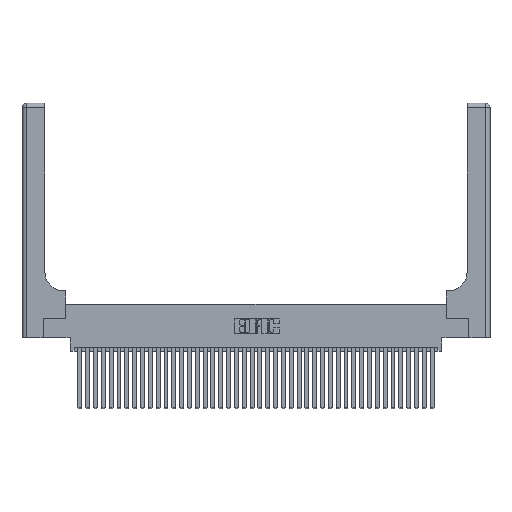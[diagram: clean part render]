
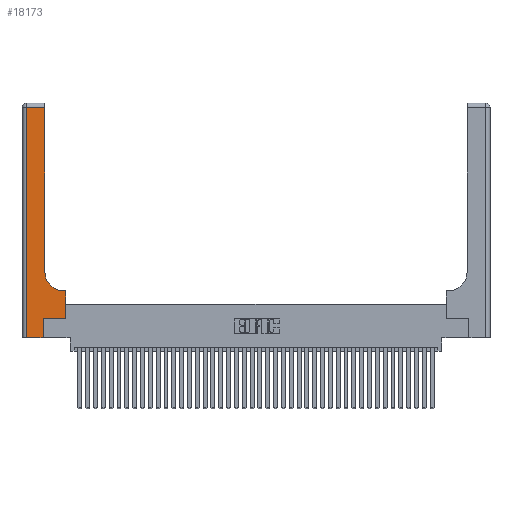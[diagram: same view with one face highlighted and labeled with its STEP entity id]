
A CAD part, top view. The second image highlights one B-rep face of the part: STEP entity #18173.
In plain terms, the highlighted planar face has unit normal (0, 0, 1).
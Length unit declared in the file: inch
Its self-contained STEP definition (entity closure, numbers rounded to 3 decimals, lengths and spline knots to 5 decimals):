
#186 = DIRECTION ( 'NONE',  ( -1., 0., 0. ) ) ;
#487 = CARTESIAN_POINT ( 'NONE',  ( 0.2915, 2.94, 0.37 ) ) ;
#1259 = VECTOR ( 'NONE', #11023, 39.37008 ) ;
#1496 = CARTESIAN_POINT ( 'NONE',  ( 0.2915, 0.6, 0.37 ) ) ;
#1696 = ORIENTED_EDGE ( 'NONE', *, *, #18250, .T. ) ;
#3113 = VECTOR ( 'NONE', #39461, 39.37008 ) ;
#3179 = VERTEX_POINT ( 'NONE', #7423 ) ;
#3605 = CARTESIAN_POINT ( 'NONE',  ( 0., 2.94, 0.37 ) ) ;
#3863 = LINE ( 'NONE', #4977, #11738 ) ;
#4977 = CARTESIAN_POINT ( 'NONE',  ( 0.269, 0., 0.37 ) ) ;
#5145 = CARTESIAN_POINT ( 'NONE',  ( 0.269, 0., 0.37 ) ) ;
#5342 = CARTESIAN_POINT ( 'NONE',  ( 0.5585, 0.6, 0.37 ) ) ;
#5347 = VERTEX_POINT ( 'NONE', #36318 ) ;
#5669 = AXIS2_PLACEMENT_3D ( 'NONE', #19370, #12613, #28831 ) ;
#6609 = DIRECTION ( 'NONE',  ( 1., 0., 0. ) ) ;
#6881 = EDGE_CURVE ( 'NONE', #18473, #3179, #17303, .T. ) ;
#7340 = DIRECTION ( 'NONE',  ( 0., 1., 0. ) ) ;
#7350 = CARTESIAN_POINT ( 'NONE',  ( 0.06, 0., 0.37 ) ) ;
#7379 = CARTESIAN_POINT ( 'NONE',  ( 0.269, 0.25, 0.37 ) ) ;
#7423 = CARTESIAN_POINT ( 'NONE',  ( 0.5585, 0.25, 0.37 ) ) ;
#7628 = LINE ( 'NONE', #20832, #1259 ) ;
#7651 = DIRECTION ( 'NONE',  ( -1., 0., 0. ) ) ;
#8691 = ORIENTED_EDGE ( 'NONE', *, *, #23717, .T. ) ;
#9276 = ORIENTED_EDGE ( 'NONE', *, *, #30700, .T. ) ;
#10074 = ORIENTED_EDGE ( 'NONE', *, *, #35673, .T. ) ;
#10418 = EDGE_CURVE ( 'NONE', #5347, #30091, #19986, .T. ) ;
#11023 = DIRECTION ( 'NONE',  ( 1., 0., 0. ) ) ;
#11505 = LINE ( 'NONE', #1496, #15518 ) ;
#11738 = VECTOR ( 'NONE', #36791, 39.37008 ) ;
#12613 = DIRECTION ( 'NONE',  ( 0., 0., -1. ) ) ;
#14313 = VECTOR ( 'NONE', #186, 39.37008 ) ;
#14418 = VERTEX_POINT ( 'NONE', #25657 ) ;
#15518 = VECTOR ( 'NONE', #7651, 39.37008 ) ;
#15998 = CARTESIAN_POINT ( 'NONE',  ( 0.269, 0.25, 0.37 ) ) ;
#17303 = LINE ( 'NONE', #15998, #22685 ) ;
#17539 = CARTESIAN_POINT ( 'NONE',  ( 0.2915, 0.85, 0.37 ) ) ;
#18173 = ADVANCED_FACE ( 'NONE', ( #25512 ), #30043, .F. ) ;
#18250 = EDGE_CURVE ( 'NONE', #36954, #18473, #3863, .T. ) ;
#18264 = LINE ( 'NONE', #3605, #14313 ) ;
#18473 = VERTEX_POINT ( 'NONE', #7379 ) ;
#18746 = EDGE_LOOP ( 'NONE', ( #9276, #8691, #24765, #40462, #1696, #39995, #23211, #10074, #25572 ) ) ;
#19227 = AXIS2_PLACEMENT_3D ( 'NONE', #33217, #23860, #27174 ) ;
#19370 = CARTESIAN_POINT ( 'NONE',  ( 0.5415, 0.85, 0.37 ) ) ;
#19986 = CIRCLE ( 'NONE', #5669, 0.25 ) ;
#20832 = CARTESIAN_POINT ( 'NONE',  ( 0., 0., 0.37 ) ) ;
#22685 = VECTOR ( 'NONE', #6609, 39.37008 ) ;
#23075 = CARTESIAN_POINT ( 'NONE',  ( 0.5585, 0.25, 0.37 ) ) ;
#23211 = ORIENTED_EDGE ( 'NONE', *, *, #25624, .T. ) ;
#23504 = CARTESIAN_POINT ( 'NONE',  ( 0.06, 3., 0.37 ) ) ;
#23717 = EDGE_CURVE ( 'NONE', #25601, #14418, #18264, .T. ) ;
#23860 = DIRECTION ( 'NONE',  ( 0., 0., -1. ) ) ;
#24513 = VERTEX_POINT ( 'NONE', #7350 ) ;
#24765 = ORIENTED_EDGE ( 'NONE', *, *, #40369, .T. ) ;
#25512 = FACE_OUTER_BOUND ( 'NONE', #18746, .T. ) ;
#25572 = ORIENTED_EDGE ( 'NONE', *, *, #10418, .T. ) ;
#25601 = VERTEX_POINT ( 'NONE', #487 ) ;
#25624 = EDGE_CURVE ( 'NONE', #3179, #32181, #37774, .T. ) ;
#25657 = CARTESIAN_POINT ( 'NONE',  ( 0.06, 2.94, 0.37 ) ) ;
#26481 = EDGE_CURVE ( 'NONE', #24513, #36954, #7628, .T. ) ;
#27087 = LINE ( 'NONE', #39899, #39395 ) ;
#27174 = DIRECTION ( 'NONE',  ( -1., 0., 0. ) ) ;
#28831 = DIRECTION ( 'NONE',  ( 1., 0., 0. ) ) ;
#30043 = PLANE ( 'NONE',  #19227 ) ;
#30091 = VERTEX_POINT ( 'NONE', #17539 ) ;
#30362 = VECTOR ( 'NONE', #7340, 39.37008 ) ;
#30700 = EDGE_CURVE ( 'NONE', #30091, #25601, #27087, .T. ) ;
#31172 = LINE ( 'NONE', #23504, #3113 ) ;
#32181 = VERTEX_POINT ( 'NONE', #5342 ) ;
#33217 = CARTESIAN_POINT ( 'NONE',  ( 0., 3., 0.37 ) ) ;
#35673 = EDGE_CURVE ( 'NONE', #32181, #5347, #11505, .T. ) ;
#36318 = CARTESIAN_POINT ( 'NONE',  ( 0.5415, 0.6, 0.37 ) ) ;
#36791 = DIRECTION ( 'NONE',  ( 0., 1., 0. ) ) ;
#36954 = VERTEX_POINT ( 'NONE', #5145 ) ;
#37774 = LINE ( 'NONE', #23075, #30362 ) ;
#39366 = DIRECTION ( 'NONE',  ( 0., 1., 0. ) ) ;
#39395 = VECTOR ( 'NONE', #39366, 39.37008 ) ;
#39461 = DIRECTION ( 'NONE',  ( 0., -1., 0. ) ) ;
#39899 = CARTESIAN_POINT ( 'NONE',  ( 0.2915, 3., 0.37 ) ) ;
#39995 = ORIENTED_EDGE ( 'NONE', *, *, #6881, .T. ) ;
#40369 = EDGE_CURVE ( 'NONE', #14418, #24513, #31172, .T. ) ;
#40462 = ORIENTED_EDGE ( 'NONE', *, *, #26481, .T. ) ;
